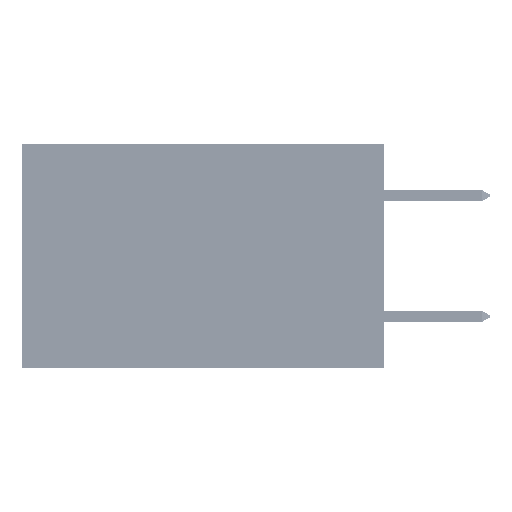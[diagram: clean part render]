
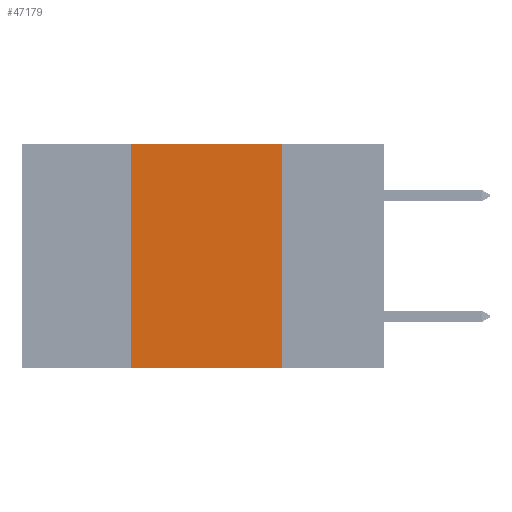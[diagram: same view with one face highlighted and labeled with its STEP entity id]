
A CAD part, left-side view. The second image highlights one B-rep face of the part: STEP entity #47179.
In plain terms, the highlighted planar face has unit normal (-1, 0, 0).
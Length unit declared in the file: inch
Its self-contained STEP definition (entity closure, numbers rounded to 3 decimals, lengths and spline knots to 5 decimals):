
#1024 = ORIENTED_EDGE ( 'NONE', *, *, #49054, .F. ) ;
#1268 = VERTEX_POINT ( 'NONE', #37004 ) ;
#3090 = DIRECTION ( 'NONE',  ( 0., 0., -1. ) ) ;
#3592 = VECTOR ( 'NONE', #26629, 39.37008 ) ;
#5447 = VERTEX_POINT ( 'NONE', #48175 ) ;
#11284 = LINE ( 'NONE', #37206, #31340 ) ;
#14280 = DIRECTION ( 'NONE',  ( 0., -1., 0. ) ) ;
#15615 = LINE ( 'NONE', #34256, #35689 ) ;
#19061 = PLANE ( 'NONE',  #21427 ) ;
#19508 = CARTESIAN_POINT ( 'NONE',  ( 0., 0.42, -0.37 ) ) ;
#21255 = DIRECTION ( 'NONE',  ( 0., -1., 0. ) ) ;
#21427 = AXIS2_PLACEMENT_3D ( 'NONE', #51150, #27085, #3090 ) ;
#22755 = VERTEX_POINT ( 'NONE', #19508 ) ;
#24925 = LINE ( 'NONE', #46633, #3592 ) ;
#25365 = LINE ( 'NONE', #29134, #36044 ) ;
#26629 = DIRECTION ( 'NONE',  ( 0., 0., 1. ) ) ;
#27085 = DIRECTION ( 'NONE',  ( 1., 0., 0. ) ) ;
#27480 = EDGE_LOOP ( 'NONE', ( #51763, #31006, #1024, #31665 ) ) ;
#29134 = CARTESIAN_POINT ( 'NONE',  ( 0., 0.17, 0. ) ) ;
#31006 = ORIENTED_EDGE ( 'NONE', *, *, #34848, .F. ) ;
#31219 = EDGE_CURVE ( 'NONE', #22755, #47091, #11284, .T. ) ;
#31340 = VECTOR ( 'NONE', #21255, 39.37008 ) ;
#31665 = ORIENTED_EDGE ( 'NONE', *, *, #31219, .T. ) ;
#34256 = CARTESIAN_POINT ( 'NONE',  ( 0., 0.6, 0. ) ) ;
#34848 = EDGE_CURVE ( 'NONE', #1268, #5447, #15615, .T. ) ;
#35689 = VECTOR ( 'NONE', #14280, 39.37008 ) ;
#36044 = VECTOR ( 'NONE', #37195, 39.37008 ) ;
#37004 = CARTESIAN_POINT ( 'NONE',  ( 0., 0.42, 0. ) ) ;
#37195 = DIRECTION ( 'NONE',  ( 0., 0., -1. ) ) ;
#37206 = CARTESIAN_POINT ( 'NONE',  ( 0., 0.6, -0.37 ) ) ;
#37282 = EDGE_CURVE ( 'NONE', #5447, #47091, #25365, .T. ) ;
#38679 = CARTESIAN_POINT ( 'NONE',  ( 0., 0.17, -0.37 ) ) ;
#42446 = FACE_OUTER_BOUND ( 'NONE', #27480, .T. ) ;
#46633 = CARTESIAN_POINT ( 'NONE',  ( 0., 0.42, 0. ) ) ;
#47091 = VERTEX_POINT ( 'NONE', #38679 ) ;
#47179 = ADVANCED_FACE ( 'NONE', ( #42446 ), #19061, .F. ) ;
#48175 = CARTESIAN_POINT ( 'NONE',  ( 0., 0.17, 0. ) ) ;
#49054 = EDGE_CURVE ( 'NONE', #22755, #1268, #24925, .T. ) ;
#51150 = CARTESIAN_POINT ( 'NONE',  ( 0., 0.6, 0. ) ) ;
#51763 = ORIENTED_EDGE ( 'NONE', *, *, #37282, .F. ) ;
